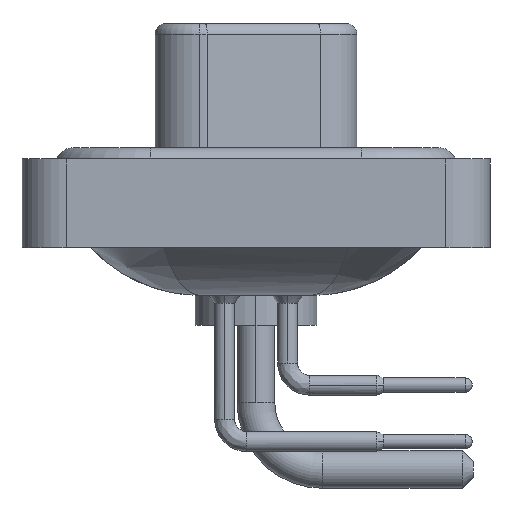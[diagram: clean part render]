
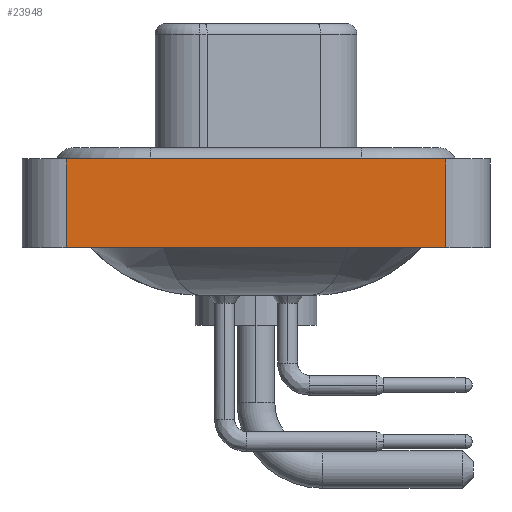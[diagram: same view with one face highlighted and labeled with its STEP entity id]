
A CAD part, left-side view. The second image highlights one B-rep face of the part: STEP entity #23948.
In plain terms, the highlighted planar face has unit normal (-1, 0, 0).
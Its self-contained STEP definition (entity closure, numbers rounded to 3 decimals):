
#3 = LINE ( 'NONE', #15578, #13361 ) ;
#394 = VERTEX_POINT ( 'NONE', #10929 ) ;
#1122 = DIRECTION ( 'NONE',  ( 0., 0., 1. ) ) ;
#1180 = EDGE_CURVE ( 'NONE', #4910, #10507, #17244, .T. ) ;
#1365 = VECTOR ( 'NONE', #6876, 1000. ) ;
#1829 = DIRECTION ( 'NONE',  ( 0., 0., 1. ) ) ;
#1904 = CARTESIAN_POINT ( 'NONE',  ( -7.3, -8.55, 0.4 ) ) ;
#2008 = CARTESIAN_POINT ( 'NONE',  ( -7.3, -8.55, 0.4 ) ) ;
#4021 = VECTOR ( 'NONE', #1122, 1000. ) ;
#4543 = DIRECTION ( 'NONE',  ( 0., 0., 1. ) ) ;
#4910 = VERTEX_POINT ( 'NONE', #8312 ) ;
#5582 = VECTOR ( 'NONE', #7805, 1000. ) ;
#5697 = EDGE_CURVE ( 'NONE', #16629, #394, #3, .T. ) ;
#6876 = DIRECTION ( 'NONE',  ( 0., -1., 0. ) ) ;
#7805 = DIRECTION ( 'NONE',  ( 0., -1., 0. ) ) ;
#8312 = CARTESIAN_POINT ( 'NONE',  ( -7.3, -8.55, -3.6 ) ) ;
#10507 = VERTEX_POINT ( 'NONE', #2008 ) ;
#10929 = CARTESIAN_POINT ( 'NONE',  ( -7.3, 8.55, 0.4 ) ) ;
#11090 = CARTESIAN_POINT ( 'NONE',  ( -7.3, -8.55, -3.6 ) ) ;
#12671 = CARTESIAN_POINT ( 'NONE',  ( -7.3, -8.55, -3.6 ) ) ;
#13294 = ORIENTED_EDGE ( 'NONE', *, *, #1180, .T. ) ;
#13361 = VECTOR ( 'NONE', #1829, 1000. ) ;
#14152 = ORIENTED_EDGE ( 'NONE', *, *, #18787, .F. ) ;
#14363 = PLANE ( 'NONE',  #16935 ) ;
#15578 = CARTESIAN_POINT ( 'NONE',  ( -7.3, 8.55, -3.6 ) ) ;
#15915 = EDGE_CURVE ( 'NONE', #16629, #4910, #22778, .T. ) ;
#16629 = VERTEX_POINT ( 'NONE', #21726 ) ;
#16732 = DIRECTION ( 'NONE',  ( -1., 0., 0. ) ) ;
#16935 = AXIS2_PLACEMENT_3D ( 'NONE', #12671, #16732, #4543 ) ;
#17244 = LINE ( 'NONE', #11090, #4021 ) ;
#18474 = FACE_OUTER_BOUND ( 'NONE', #19660, .T. ) ;
#18787 = EDGE_CURVE ( 'NONE', #394, #10507, #21721, .T. ) ;
#19660 = EDGE_LOOP ( 'NONE', ( #13294, #14152, #21993, #20673 ) ) ;
#20673 = ORIENTED_EDGE ( 'NONE', *, *, #15915, .T. ) ;
#21721 = LINE ( 'NONE', #1904, #5582 ) ;
#21726 = CARTESIAN_POINT ( 'NONE',  ( -7.3, 8.55, -3.6 ) ) ;
#21993 = ORIENTED_EDGE ( 'NONE', *, *, #5697, .F. ) ;
#22778 = LINE ( 'NONE', #24869, #1365 ) ;
#23948 = ADVANCED_FACE ( 'NONE', ( #18474 ), #14363, .T. ) ;
#24869 = CARTESIAN_POINT ( 'NONE',  ( -7.3, -8.55, -3.6 ) ) ;
